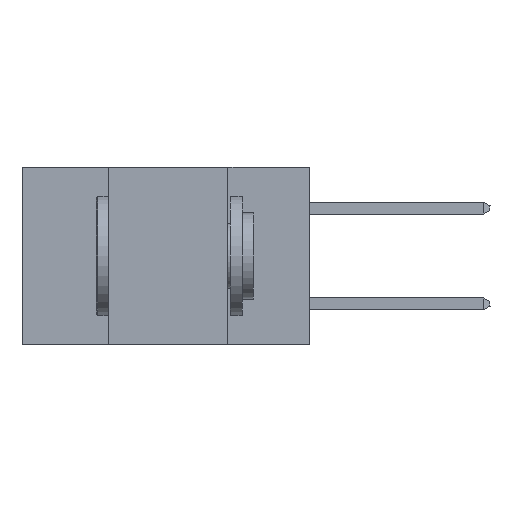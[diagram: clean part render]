
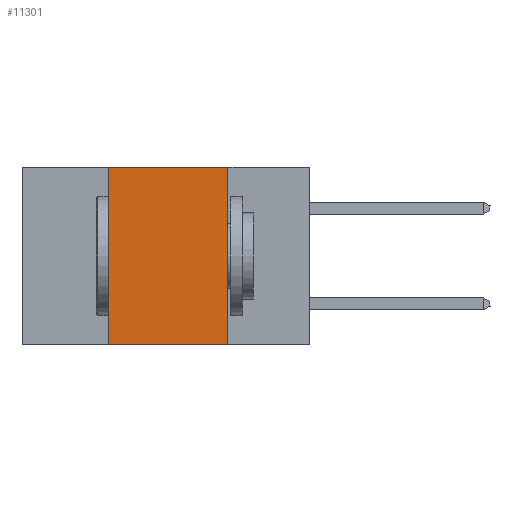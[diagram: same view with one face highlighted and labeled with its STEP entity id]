
A CAD part, left-side view. The second image highlights one B-rep face of the part: STEP entity #11301.
In plain terms, the highlighted planar face has unit normal (-1, 0, 0).
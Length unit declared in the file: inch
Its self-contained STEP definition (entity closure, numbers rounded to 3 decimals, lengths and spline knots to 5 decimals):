
#138 = VERTEX_POINT ( 'NONE', #3501 ) ;
#527 = AXIS2_PLACEMENT_3D ( 'NONE', #11804, #5906, #26605 ) ;
#774 = VERTEX_POINT ( 'NONE', #10450 ) ;
#915 = ORIENTED_EDGE ( 'NONE', *, *, #16877, .T. ) ;
#1400 = VERTEX_POINT ( 'NONE', #6218 ) ;
#3501 = CARTESIAN_POINT ( 'NONE',  ( 0., 0.17, 0. ) ) ;
#5906 = DIRECTION ( 'NONE',  ( 1., 0., 0. ) ) ;
#5959 = EDGE_CURVE ( 'NONE', #138, #23238, #35426, .T. ) ;
#6218 = CARTESIAN_POINT ( 'NONE',  ( 0., 0.42, 0. ) ) ;
#7766 = LINE ( 'NONE', #9696, #15663 ) ;
#9696 = CARTESIAN_POINT ( 'NONE',  ( 0., 0.42, 0. ) ) ;
#10336 = CARTESIAN_POINT ( 'NONE',  ( 0., 0.6, 0. ) ) ;
#10450 = CARTESIAN_POINT ( 'NONE',  ( 0., 0.42, -0.37 ) ) ;
#11301 = ADVANCED_FACE ( 'NONE', ( #23958 ), #38243, .F. ) ;
#11493 = EDGE_CURVE ( 'NONE', #774, #1400, #7766, .T. ) ;
#11522 = LINE ( 'NONE', #10336, #33108 ) ;
#11804 = CARTESIAN_POINT ( 'NONE',  ( 0., 0.6, 0. ) ) ;
#11972 = VECTOR ( 'NONE', #14741, 39.37008 ) ;
#13321 = DIRECTION ( 'NONE',  ( 0., -1., 0. ) ) ;
#14741 = DIRECTION ( 'NONE',  ( 0., 0., -1. ) ) ;
#15663 = VECTOR ( 'NONE', #33239, 39.37008 ) ;
#16877 = EDGE_CURVE ( 'NONE', #774, #23238, #25382, .T. ) ;
#17711 = EDGE_CURVE ( 'NONE', #1400, #138, #11522, .T. ) ;
#21299 = DIRECTION ( 'NONE',  ( 0., -1., 0. ) ) ;
#21440 = EDGE_LOOP ( 'NONE', ( #26043, #34757, #21833, #915 ) ) ;
#21833 = ORIENTED_EDGE ( 'NONE', *, *, #11493, .F. ) ;
#23238 = VERTEX_POINT ( 'NONE', #34078 ) ;
#23958 = FACE_OUTER_BOUND ( 'NONE', #21440, .T. ) ;
#24449 = VECTOR ( 'NONE', #21299, 39.37008 ) ;
#25382 = LINE ( 'NONE', #27167, #24449 ) ;
#26043 = ORIENTED_EDGE ( 'NONE', *, *, #5959, .F. ) ;
#26574 = CARTESIAN_POINT ( 'NONE',  ( 0., 0.17, 0. ) ) ;
#26605 = DIRECTION ( 'NONE',  ( 0., 0., -1. ) ) ;
#27167 = CARTESIAN_POINT ( 'NONE',  ( 0., 0.6, -0.37 ) ) ;
#33108 = VECTOR ( 'NONE', #13321, 39.37008 ) ;
#33239 = DIRECTION ( 'NONE',  ( 0., 0., 1. ) ) ;
#34078 = CARTESIAN_POINT ( 'NONE',  ( 0., 0.17, -0.37 ) ) ;
#34757 = ORIENTED_EDGE ( 'NONE', *, *, #17711, .F. ) ;
#35426 = LINE ( 'NONE', #26574, #11972 ) ;
#38243 = PLANE ( 'NONE',  #527 ) ;
